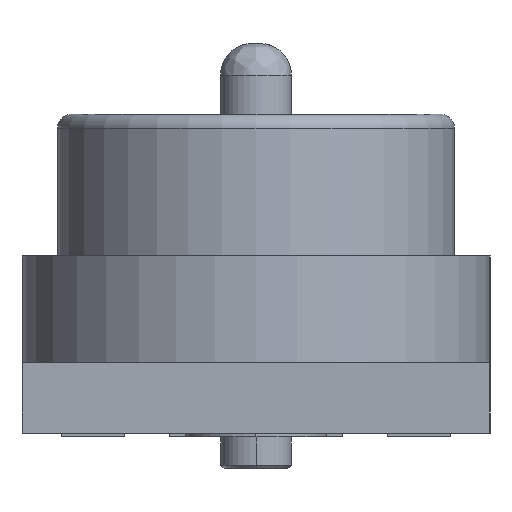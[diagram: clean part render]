
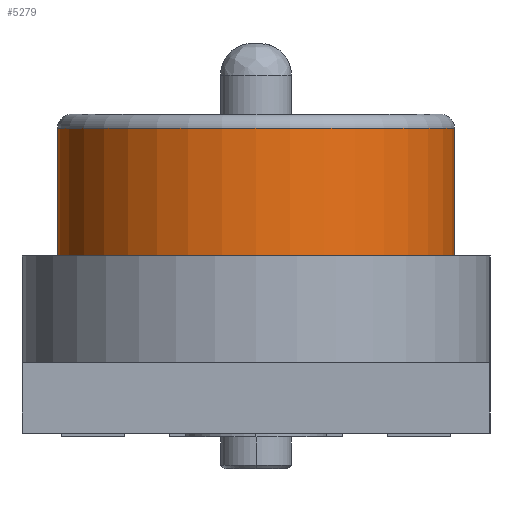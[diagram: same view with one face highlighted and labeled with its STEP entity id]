
A CAD part, left-side view. The second image highlights one B-rep face of the part: STEP entity #5279.
In plain terms, the highlighted cylindrical face has radius 2.8 mm (diameter 5.6 mm), a partial arc.
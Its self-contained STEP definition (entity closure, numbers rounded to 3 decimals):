
#418 = EDGE_CURVE ( 'NONE', #7693, #3869, #1306, .T. ) ;
#479 = ORIENTED_EDGE ( 'NONE', *, *, #418, .F. ) ;
#966 = ORIENTED_EDGE ( 'NONE', *, *, #4531, .F. ) ;
#968 = AXIS2_PLACEMENT_3D ( 'NONE', #2974, #2279, #1768 ) ;
#1306 = LINE ( 'NONE', #7465, #3689 ) ;
#1476 = CARTESIAN_POINT ( 'NONE',  ( -8.63, 0., 1.8 ) ) ;
#1555 = DIRECTION ( 'NONE',  ( 0., 0., -1. ) ) ;
#1768 = DIRECTION ( 'NONE',  ( 1., 0., 0. ) ) ;
#1852 = AXIS2_PLACEMENT_3D ( 'NONE', #4115, #2933, #4674 ) ;
#2167 = EDGE_LOOP ( 'NONE', ( #479, #2298, #966, #3479 ) ) ;
#2255 = LINE ( 'NONE', #6428, #5402 ) ;
#2279 = DIRECTION ( 'NONE',  ( 0., 0., 1. ) ) ;
#2298 = ORIENTED_EDGE ( 'NONE', *, *, #6805, .T. ) ;
#2406 = CYLINDRICAL_SURFACE ( 'NONE', #968, 2.8 ) ;
#2414 = CARTESIAN_POINT ( 'NONE',  ( -8.63, -2.8, 1.8 ) ) ;
#2933 = DIRECTION ( 'NONE',  ( 0., 0., 1. ) ) ;
#2974 = CARTESIAN_POINT ( 'NONE',  ( -8.63, 0., -0.036 ) ) ;
#3479 = ORIENTED_EDGE ( 'NONE', *, *, #5214, .T. ) ;
#3523 = CARTESIAN_POINT ( 'NONE',  ( -8.63, -2.8, 0. ) ) ;
#3665 = CARTESIAN_POINT ( 'NONE',  ( -8.63, 2.8, 1.8 ) ) ;
#3689 = VECTOR ( 'NONE', #5606, 1000. ) ;
#3869 = VERTEX_POINT ( 'NONE', #3665 ) ;
#4044 = AXIS2_PLACEMENT_3D ( 'NONE', #1476, #1555, #6374 ) ;
#4115 = CARTESIAN_POINT ( 'NONE',  ( -8.63, 0., 0. ) ) ;
#4531 = EDGE_CURVE ( 'NONE', #7620, #7266, #2255, .T. ) ;
#4674 = DIRECTION ( 'NONE',  ( 0., 1., 0. ) ) ;
#5214 = EDGE_CURVE ( 'NONE', #7620, #3869, #5601, .T. ) ;
#5279 = ADVANCED_FACE ( 'NONE', ( #7930 ), #2406, .T. ) ;
#5354 = CIRCLE ( 'NONE', #1852, 2.8 ) ;
#5402 = VECTOR ( 'NONE', #7189, 1000. ) ;
#5601 = CIRCLE ( 'NONE', #4044, 2.8 ) ;
#5606 = DIRECTION ( 'NONE',  ( 0., 0., 1. ) ) ;
#6374 = DIRECTION ( 'NONE',  ( -0.013, 1., 0. ) ) ;
#6428 = CARTESIAN_POINT ( 'NONE',  ( -8.63, -2.8, 1.8 ) ) ;
#6805 = EDGE_CURVE ( 'NONE', #7693, #7266, #5354, .T. ) ;
#7189 = DIRECTION ( 'NONE',  ( 0., 0., -1. ) ) ;
#7266 = VERTEX_POINT ( 'NONE', #3523 ) ;
#7465 = CARTESIAN_POINT ( 'NONE',  ( -8.63, 2.8, 0. ) ) ;
#7620 = VERTEX_POINT ( 'NONE', #2414 ) ;
#7693 = VERTEX_POINT ( 'NONE', #7941 ) ;
#7930 = FACE_OUTER_BOUND ( 'NONE', #2167, .T. ) ;
#7941 = CARTESIAN_POINT ( 'NONE',  ( -8.63, 2.8, 0. ) ) ;
